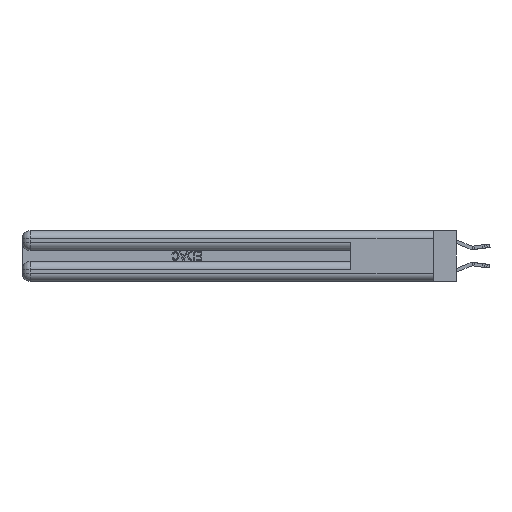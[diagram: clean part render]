
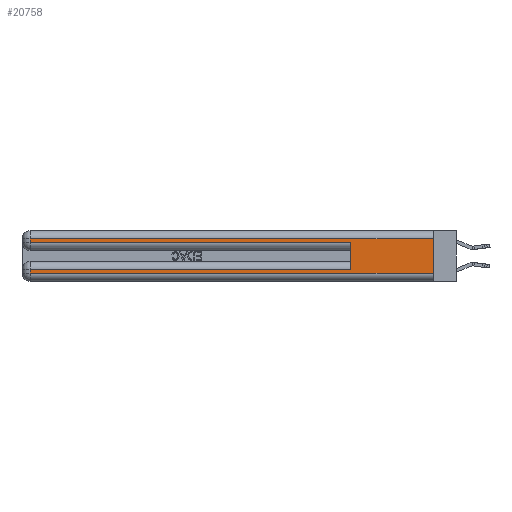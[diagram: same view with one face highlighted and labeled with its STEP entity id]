
A CAD part, left-side view. The second image highlights one B-rep face of the part: STEP entity #20758.
In plain terms, the highlighted planar face has unit normal (-1, 0, 0).
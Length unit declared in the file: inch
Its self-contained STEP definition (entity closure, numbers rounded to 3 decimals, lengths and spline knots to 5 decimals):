
#117 = CARTESIAN_POINT ( 'NONE',  ( 0., 2.94, 0.37 ) ) ;
#906 = DIRECTION ( 'NONE',  ( 1., 0., 0. ) ) ;
#1394 = VERTEX_POINT ( 'NONE', #9639 ) ;
#1510 = LINE ( 'NONE', #11710, #27212 ) ;
#1717 = DIRECTION ( 'NONE',  ( 0., -1., 0. ) ) ;
#1794 = CARTESIAN_POINT ( 'NONE',  ( 0., 0., 0.285 ) ) ;
#1820 = VECTOR ( 'NONE', #23146, 39.37008 ) ;
#2340 = EDGE_CURVE ( 'NONE', #2967, #11187, #1510, .T. ) ;
#2536 = DIRECTION ( 'NONE',  ( 0., 0., 1. ) ) ;
#2967 = VERTEX_POINT ( 'NONE', #23309 ) ;
#3155 = ORIENTED_EDGE ( 'NONE', *, *, #23555, .T. ) ;
#3239 = CARTESIAN_POINT ( 'NONE',  ( 0., 0.6, 0.285 ) ) ;
#3750 = AXIS2_PLACEMENT_3D ( 'NONE', #8598, #906, #29141 ) ;
#3894 = EDGE_CURVE ( 'NONE', #2967, #13971, #28370, .T. ) ;
#4519 = DIRECTION ( 'NONE',  ( 0., 0., -1. ) ) ;
#5655 = CARTESIAN_POINT ( 'NONE',  ( 0., 0., 0.31 ) ) ;
#6022 = CARTESIAN_POINT ( 'NONE',  ( 0., 2.94, 0.31 ) ) ;
#7154 = LINE ( 'NONE', #117, #1820 ) ;
#7974 = EDGE_CURVE ( 'NONE', #17511, #15050, #20309, .T. ) ;
#8198 = LINE ( 'NONE', #15236, #26358 ) ;
#8598 = CARTESIAN_POINT ( 'NONE',  ( 0., 0., 0.37 ) ) ;
#8889 = CARTESIAN_POINT ( 'NONE',  ( 0., 2.94, 0.085 ) ) ;
#8922 = ORIENTED_EDGE ( 'NONE', *, *, #17533, .T. ) ;
#9639 = CARTESIAN_POINT ( 'NONE',  ( 0., 2.94, 0.06 ) ) ;
#10030 = EDGE_LOOP ( 'NONE', ( #32628, #12137, #8922, #32895, #14451, #18232, #10078, #3155 ) ) ;
#10078 = ORIENTED_EDGE ( 'NONE', *, *, #32459, .T. ) ;
#10112 = EDGE_CURVE ( 'NONE', #17511, #26383, #8198, .T. ) ;
#11187 = VERTEX_POINT ( 'NONE', #17406 ) ;
#11691 = VECTOR ( 'NONE', #17618, 39.37008 ) ;
#11710 = CARTESIAN_POINT ( 'NONE',  ( 0., 0., 0.37 ) ) ;
#12045 = CARTESIAN_POINT ( 'NONE',  ( 0., 2.94, 0.285 ) ) ;
#12137 = ORIENTED_EDGE ( 'NONE', *, *, #3894, .T. ) ;
#13971 = VERTEX_POINT ( 'NONE', #6022 ) ;
#14451 = ORIENTED_EDGE ( 'NONE', *, *, #10112, .F. ) ;
#14505 = DIRECTION ( 'NONE',  ( 0., -1., 0. ) ) ;
#14510 = VECTOR ( 'NONE', #14505, 39.37008 ) ;
#14628 = LINE ( 'NONE', #24641, #11691 ) ;
#14752 = LINE ( 'NONE', #27271, #19636 ) ;
#15050 = VERTEX_POINT ( 'NONE', #8889 ) ;
#15236 = CARTESIAN_POINT ( 'NONE',  ( 0., 0.6, 0.145 ) ) ;
#15477 = VECTOR ( 'NONE', #25811, 39.37008 ) ;
#17005 = LINE ( 'NONE', #1794, #14510 ) ;
#17133 = CARTESIAN_POINT ( 'NONE',  ( 0., 0.6, 0.085 ) ) ;
#17406 = CARTESIAN_POINT ( 'NONE',  ( 0., 0., 0.06 ) ) ;
#17511 = VERTEX_POINT ( 'NONE', #17133 ) ;
#17533 = EDGE_CURVE ( 'NONE', #13971, #24036, #14628, .T. ) ;
#17618 = DIRECTION ( 'NONE',  ( 0., 0., -1. ) ) ;
#18232 = ORIENTED_EDGE ( 'NONE', *, *, #7974, .T. ) ;
#19636 = VECTOR ( 'NONE', #1717, 39.37008 ) ;
#20309 = LINE ( 'NONE', #28158, #15477 ) ;
#20359 = DIRECTION ( 'NONE',  ( 0., 1., 0. ) ) ;
#20758 = ADVANCED_FACE ( 'NONE', ( #23616 ), #21282, .F. ) ;
#21282 = PLANE ( 'NONE',  #3750 ) ;
#22527 = EDGE_CURVE ( 'NONE', #24036, #26383, #17005, .T. ) ;
#23146 = DIRECTION ( 'NONE',  ( 0., 0., -1. ) ) ;
#23309 = CARTESIAN_POINT ( 'NONE',  ( 0., 0., 0.31 ) ) ;
#23555 = EDGE_CURVE ( 'NONE', #1394, #11187, #14752, .T. ) ;
#23616 = FACE_OUTER_BOUND ( 'NONE', #10030, .T. ) ;
#24036 = VERTEX_POINT ( 'NONE', #12045 ) ;
#24641 = CARTESIAN_POINT ( 'NONE',  ( 0., 2.94, 0.37 ) ) ;
#25811 = DIRECTION ( 'NONE',  ( 0., 1., 0. ) ) ;
#25881 = VECTOR ( 'NONE', #20359, 39.37008 ) ;
#26358 = VECTOR ( 'NONE', #2536, 39.37008 ) ;
#26383 = VERTEX_POINT ( 'NONE', #3239 ) ;
#27212 = VECTOR ( 'NONE', #4519, 39.37008 ) ;
#27271 = CARTESIAN_POINT ( 'NONE',  ( 0., 0., 0.06 ) ) ;
#28158 = CARTESIAN_POINT ( 'NONE',  ( 0., 0., 0.085 ) ) ;
#28370 = LINE ( 'NONE', #5655, #25881 ) ;
#29141 = DIRECTION ( 'NONE',  ( 0., 0., -1. ) ) ;
#32459 = EDGE_CURVE ( 'NONE', #15050, #1394, #7154, .T. ) ;
#32628 = ORIENTED_EDGE ( 'NONE', *, *, #2340, .F. ) ;
#32895 = ORIENTED_EDGE ( 'NONE', *, *, #22527, .T. ) ;
